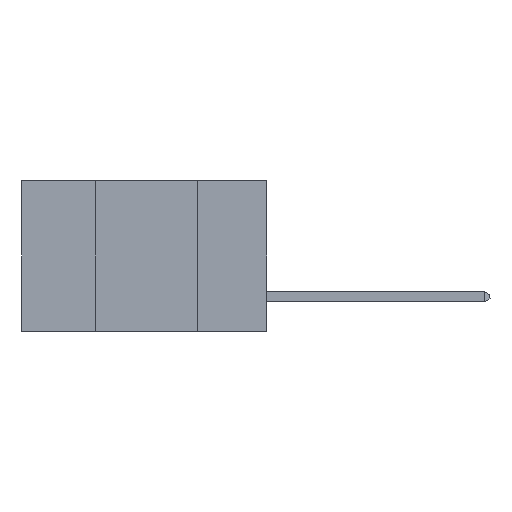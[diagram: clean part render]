
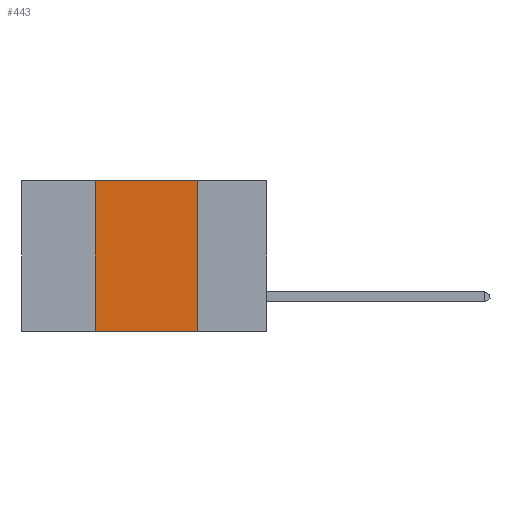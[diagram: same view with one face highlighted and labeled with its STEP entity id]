
A CAD part, left-side view. The second image highlights one B-rep face of the part: STEP entity #443.
In plain terms, the highlighted planar face has unit normal (-1, 0, 0).
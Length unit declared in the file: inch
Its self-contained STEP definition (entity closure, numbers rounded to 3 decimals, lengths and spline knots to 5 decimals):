
#235 = ORIENTED_EDGE ( 'NONE', *, *, #2248, .F. ) ;
#377 = VECTOR ( 'NONE', #5635, 39.37008 ) ;
#443 = ADVANCED_FACE ( 'NONE', ( #14266 ), #1769, .F. ) ;
#611 = DIRECTION ( 'NONE',  ( 0., 0., -1. ) ) ;
#622 = DIRECTION ( 'NONE',  ( 1., 0., 0. ) ) ;
#649 = CARTESIAN_POINT ( 'NONE',  ( 0., 0.6, 0. ) ) ;
#1235 = VECTOR ( 'NONE', #11435, 39.37008 ) ;
#1636 = VECTOR ( 'NONE', #1664, 39.37008 ) ;
#1664 = DIRECTION ( 'NONE',  ( 0., 0., -1. ) ) ;
#1713 = VERTEX_POINT ( 'NONE', #11348 ) ;
#1769 = PLANE ( 'NONE',  #14626 ) ;
#2233 = CARTESIAN_POINT ( 'NONE',  ( 0., 0.42, -0.37 ) ) ;
#2248 = EDGE_CURVE ( 'NONE', #2703, #1713, #12921, .T. ) ;
#2703 = VERTEX_POINT ( 'NONE', #8584 ) ;
#4012 = EDGE_CURVE ( 'NONE', #1713, #14654, #12853, .T. ) ;
#4097 = CARTESIAN_POINT ( 'NONE',  ( 0., 0.42, 0. ) ) ;
#5635 = DIRECTION ( 'NONE',  ( 0., 0., 1. ) ) ;
#5807 = EDGE_LOOP ( 'NONE', ( #18558, #235, #8269, #15745 ) ) ;
#8208 = CARTESIAN_POINT ( 'NONE',  ( 0., 0.17, -0.37 ) ) ;
#8269 = ORIENTED_EDGE ( 'NONE', *, *, #16830, .F. ) ;
#8584 = CARTESIAN_POINT ( 'NONE',  ( 0., 0.42, 0. ) ) ;
#10318 = VERTEX_POINT ( 'NONE', #2233 ) ;
#10346 = DIRECTION ( 'NONE',  ( 0., -1., 0. ) ) ;
#11348 = CARTESIAN_POINT ( 'NONE',  ( 0., 0.17, 0. ) ) ;
#11435 = DIRECTION ( 'NONE',  ( 0., -1., 0. ) ) ;
#11560 = CARTESIAN_POINT ( 'NONE',  ( 0., 0.6, 0. ) ) ;
#11949 = CARTESIAN_POINT ( 'NONE',  ( 0., 0.17, 0. ) ) ;
#12170 = LINE ( 'NONE', #4097, #377 ) ;
#12853 = LINE ( 'NONE', #11949, #1636 ) ;
#12921 = LINE ( 'NONE', #11560, #1235 ) ;
#14266 = FACE_OUTER_BOUND ( 'NONE', #5807, .T. ) ;
#14528 = CARTESIAN_POINT ( 'NONE',  ( 0., 0.6, -0.37 ) ) ;
#14626 = AXIS2_PLACEMENT_3D ( 'NONE', #649, #622, #611 ) ;
#14654 = VERTEX_POINT ( 'NONE', #8208 ) ;
#14946 = EDGE_CURVE ( 'NONE', #10318, #14654, #15741, .T. ) ;
#15293 = VECTOR ( 'NONE', #10346, 39.37008 ) ;
#15741 = LINE ( 'NONE', #14528, #15293 ) ;
#15745 = ORIENTED_EDGE ( 'NONE', *, *, #14946, .T. ) ;
#16830 = EDGE_CURVE ( 'NONE', #10318, #2703, #12170, .T. ) ;
#18558 = ORIENTED_EDGE ( 'NONE', *, *, #4012, .F. ) ;
